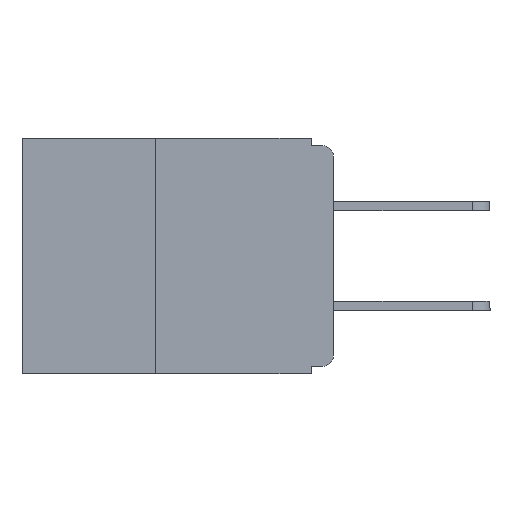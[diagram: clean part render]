
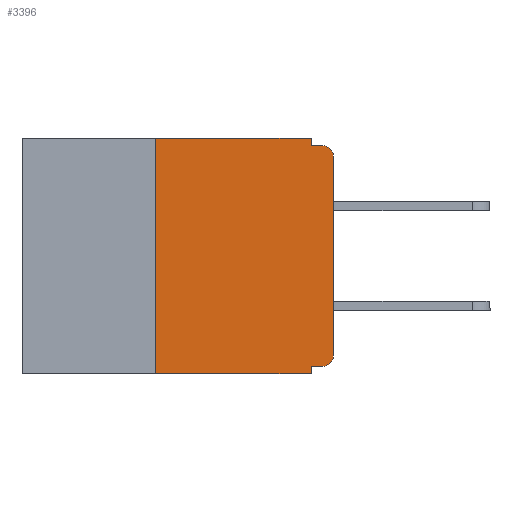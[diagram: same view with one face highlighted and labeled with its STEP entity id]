
A CAD part, left-side view. The second image highlights one B-rep face of the part: STEP entity #3396.
In plain terms, the highlighted planar face has unit normal (-1, 0, 0).
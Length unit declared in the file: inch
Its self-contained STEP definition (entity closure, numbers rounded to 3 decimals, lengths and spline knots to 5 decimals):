
#7 = CARTESIAN_POINT ( 'NONE',  ( 0., 0.25, 0. ) ) ;
#169 = VECTOR ( 'NONE', #5162, 39.37008 ) ;
#225 = VECTOR ( 'NONE', #8332, 39.37008 ) ;
#294 = ORIENTED_EDGE ( 'NONE', *, *, #13934, .F. ) ;
#478 = CARTESIAN_POINT ( 'NONE',  ( 0., 0.031, 0. ) ) ;
#554 = EDGE_CURVE ( 'NONE', #14049, #13493, #13662, .T. ) ;
#684 = CARTESIAN_POINT ( 'NONE',  ( 0., 0.031, -0.33 ) ) ;
#887 = VERTEX_POINT ( 'NONE', #15093 ) ;
#1504 = CIRCLE ( 'NONE', #10092, 0.015 ) ;
#1579 = CARTESIAN_POINT ( 'NONE',  ( 0., 0., -0.025 ) ) ;
#1770 = LINE ( 'NONE', #11985, #15132 ) ;
#1950 = CARTESIAN_POINT ( 'NONE',  ( 0., 0.015, -0.025 ) ) ;
#2188 = LINE ( 'NONE', #16063, #11401 ) ;
#2344 = CIRCLE ( 'NONE', #12177, 0.015 ) ;
#2678 = DIRECTION ( 'NONE',  ( 0., -1., 0. ) ) ;
#2908 = EDGE_CURVE ( 'NONE', #11040, #14049, #8636, .T. ) ;
#3096 = VECTOR ( 'NONE', #15936, 39.37008 ) ;
#3235 = DIRECTION ( 'NONE',  ( 0., 0., -1. ) ) ;
#3396 = ADVANCED_FACE ( 'NONE', ( #5342 ), #12169, .F. ) ;
#3614 = CARTESIAN_POINT ( 'NONE',  ( 0., 0.437, 0. ) ) ;
#3787 = VERTEX_POINT ( 'NONE', #684 ) ;
#3794 = ORIENTED_EDGE ( 'NONE', *, *, #12260, .T. ) ;
#3814 = CARTESIAN_POINT ( 'NONE',  ( 0., 0., -0.32 ) ) ;
#4270 = DIRECTION ( 'NONE',  ( 1., 0., 0. ) ) ;
#4547 = CARTESIAN_POINT ( 'NONE',  ( 0., 0.031, -0.01 ) ) ;
#4650 = ORIENTED_EDGE ( 'NONE', *, *, #2908, .F. ) ;
#4739 = DIRECTION ( 'NONE',  ( 0., 0., -1. ) ) ;
#5015 = EDGE_CURVE ( 'NONE', #6141, #5930, #2188, .T. ) ;
#5054 = VERTEX_POINT ( 'NONE', #14904 ) ;
#5162 = DIRECTION ( 'NONE',  ( 0., 1., 0. ) ) ;
#5258 = ORIENTED_EDGE ( 'NONE', *, *, #6584, .T. ) ;
#5342 = FACE_OUTER_BOUND ( 'NONE', #15418, .T. ) ;
#5930 = VERTEX_POINT ( 'NONE', #1579 ) ;
#6141 = VERTEX_POINT ( 'NONE', #11854 ) ;
#6584 = EDGE_CURVE ( 'NONE', #5054, #6141, #2344, .T. ) ;
#6851 = CARTESIAN_POINT ( 'NONE',  ( 0., 0.015, -0.01 ) ) ;
#8173 = DIRECTION ( 'NONE',  ( 0., 0., 1. ) ) ;
#8332 = DIRECTION ( 'NONE',  ( 0., 0., -1. ) ) ;
#8439 = VECTOR ( 'NONE', #12966, 39.37008 ) ;
#8636 = LINE ( 'NONE', #3614, #15000 ) ;
#8795 = CARTESIAN_POINT ( 'NONE',  ( 0., 0.031, 0. ) ) ;
#8954 = ORIENTED_EDGE ( 'NONE', *, *, #10050, .T. ) ;
#9611 = CARTESIAN_POINT ( 'NONE',  ( 0., 0., -0.01 ) ) ;
#9722 = EDGE_CURVE ( 'NONE', #13493, #14548, #10110, .T. ) ;
#9902 = LINE ( 'NONE', #14665, #225 ) ;
#9975 = ORIENTED_EDGE ( 'NONE', *, *, #15994, .F. ) ;
#10050 = EDGE_CURVE ( 'NONE', #5930, #14548, #1504, .T. ) ;
#10092 = AXIS2_PLACEMENT_3D ( 'NONE', #1950, #11098, #3235 ) ;
#10110 = LINE ( 'NONE', #9611, #3096 ) ;
#10176 = ORIENTED_EDGE ( 'NONE', *, *, #9722, .F. ) ;
#10315 = VECTOR ( 'NONE', #4739, 39.37008 ) ;
#10422 = CARTESIAN_POINT ( 'NONE',  ( 0., 0.437, -0.33 ) ) ;
#10557 = EDGE_CURVE ( 'NONE', #887, #3787, #9902, .T. ) ;
#10647 = LINE ( 'NONE', #3814, #169 ) ;
#11040 = VERTEX_POINT ( 'NONE', #7 ) ;
#11098 = DIRECTION ( 'NONE',  ( -1., 0., 0. ) ) ;
#11144 = DIRECTION ( 'NONE',  ( 0., 0., -1. ) ) ;
#11149 = DIRECTION ( 'NONE',  ( -1., 0., 0. ) ) ;
#11182 = CARTESIAN_POINT ( 'NONE',  ( 0., 0.015, -0.305 ) ) ;
#11401 = VECTOR ( 'NONE', #15942, 39.37008 ) ;
#11831 = LINE ( 'NONE', #10422, #8439 ) ;
#11854 = CARTESIAN_POINT ( 'NONE',  ( 0., 0., -0.305 ) ) ;
#11985 = CARTESIAN_POINT ( 'NONE',  ( 0., 0.25, -0.33 ) ) ;
#12169 = PLANE ( 'NONE',  #12255 ) ;
#12177 = AXIS2_PLACEMENT_3D ( 'NONE', #11182, #11149, #11144 ) ;
#12255 = AXIS2_PLACEMENT_3D ( 'NONE', #13928, #4270, #14433 ) ;
#12260 = EDGE_CURVE ( 'NONE', #16586, #3787, #11831, .T. ) ;
#12943 = CARTESIAN_POINT ( 'NONE',  ( 0., 0.25, -0.33 ) ) ;
#12966 = DIRECTION ( 'NONE',  ( 0., -1., 0. ) ) ;
#13493 = VERTEX_POINT ( 'NONE', #4547 ) ;
#13662 = LINE ( 'NONE', #8795, #10315 ) ;
#13924 = ORIENTED_EDGE ( 'NONE', *, *, #5015, .T. ) ;
#13928 = CARTESIAN_POINT ( 'NONE',  ( 0., 0.437, 0. ) ) ;
#13934 = EDGE_CURVE ( 'NONE', #16586, #11040, #1770, .T. ) ;
#14049 = VERTEX_POINT ( 'NONE', #478 ) ;
#14433 = DIRECTION ( 'NONE',  ( 0., 0., -1. ) ) ;
#14548 = VERTEX_POINT ( 'NONE', #6851 ) ;
#14665 = CARTESIAN_POINT ( 'NONE',  ( 0., 0.031, -0.33 ) ) ;
#14904 = CARTESIAN_POINT ( 'NONE',  ( 0., 0.015, -0.32 ) ) ;
#15000 = VECTOR ( 'NONE', #2678, 39.37008 ) ;
#15093 = CARTESIAN_POINT ( 'NONE',  ( 0., 0.031, -0.32 ) ) ;
#15132 = VECTOR ( 'NONE', #8173, 39.37008 ) ;
#15418 = EDGE_LOOP ( 'NONE', ( #13924, #8954, #10176, #15500, #4650, #294, #3794, #15917, #9975, #5258 ) ) ;
#15500 = ORIENTED_EDGE ( 'NONE', *, *, #554, .F. ) ;
#15917 = ORIENTED_EDGE ( 'NONE', *, *, #10557, .F. ) ;
#15936 = DIRECTION ( 'NONE',  ( 0., -1., 0. ) ) ;
#15942 = DIRECTION ( 'NONE',  ( 0., 0., 1. ) ) ;
#15994 = EDGE_CURVE ( 'NONE', #5054, #887, #10647, .T. ) ;
#16063 = CARTESIAN_POINT ( 'NONE',  ( 0., 0., 0. ) ) ;
#16586 = VERTEX_POINT ( 'NONE', #12943 ) ;
